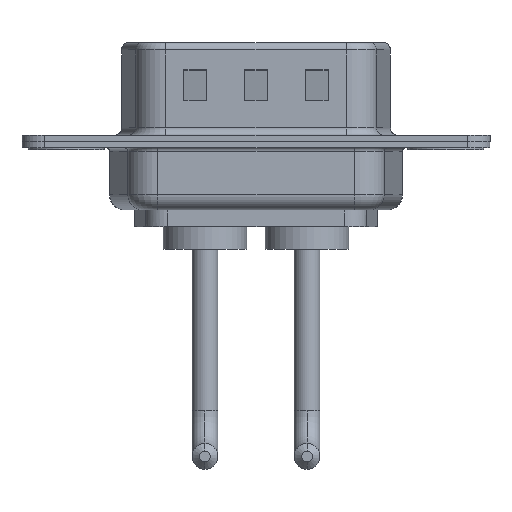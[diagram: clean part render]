
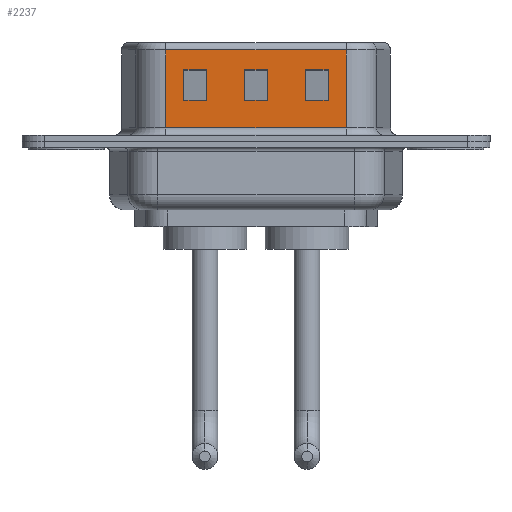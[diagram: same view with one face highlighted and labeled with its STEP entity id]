
A CAD part, front view. The second image highlights one B-rep face of the part: STEP entity #2237.
In plain terms, the highlighted planar face has unit normal (0, -1, 0).
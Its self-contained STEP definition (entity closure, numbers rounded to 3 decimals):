
#38 = VECTOR ( 'NONE', #927, 1000. ) ;
#124 = VERTEX_POINT ( 'NONE', #11989 ) ;
#233 = LINE ( 'NONE', #4109, #7689 ) ;
#274 = CARTESIAN_POINT ( 'NONE',  ( 22.451, -4.55, 2.705 ) ) ;
#290 = CARTESIAN_POINT ( 'NONE',  ( 18.451, -4.55, 6.52 ) ) ;
#459 = EDGE_CURVE ( 'NONE', #4935, #2185, #12560, .T. ) ;
#797 = VECTOR ( 'NONE', #11295, 1000. ) ;
#838 = ORIENTED_EDGE ( 'NONE', *, *, #1437, .T. ) ;
#859 = LINE ( 'NONE', #5694, #10427 ) ;
#927 = DIRECTION ( 'NONE',  ( -1., 0., 0. ) ) ;
#1058 = ORIENTED_EDGE ( 'NONE', *, *, #2612, .T. ) ;
#1204 = CARTESIAN_POINT ( 'NONE',  ( 18.451, -4.55, 6.52 ) ) ;
#1213 = DIRECTION ( 'NONE',  ( 0., 0., -1. ) ) ;
#1287 = DIRECTION ( 'NONE',  ( -1., 0., 0. ) ) ;
#1318 = VECTOR ( 'NONE', #7643, 1000. ) ;
#1386 = VECTOR ( 'NONE', #2738, 1000. ) ;
#1404 = EDGE_LOOP ( 'NONE', ( #4933, #6059, #4356, #838 ) ) ;
#1411 = EDGE_CURVE ( 'NONE', #7855, #5947, #2452, .T. ) ;
#1437 = EDGE_CURVE ( 'NONE', #5947, #4728, #233, .T. ) ;
#1714 = LINE ( 'NONE', #5466, #8401 ) ;
#1787 = CARTESIAN_POINT ( 'NONE',  ( 7.75, -4.55, 6.52 ) ) ;
#1921 = VECTOR ( 'NONE', #7525, 1000. ) ;
#1956 = ORIENTED_EDGE ( 'NONE', *, *, #8740, .T. ) ;
#2049 = CARTESIAN_POINT ( 'NONE',  ( 6.549, -4.55, 6.02 ) ) ;
#2185 = VERTEX_POINT ( 'NONE', #8154 ) ;
#2227 = CARTESIAN_POINT ( 'NONE',  ( 17.25, -4.55, 6.52 ) ) ;
#2237 = ADVANCED_FACE ( 'NONE', ( #4418, #5239, #2308, #10213 ), #10157, .F. ) ;
#2308 = FACE_BOUND ( 'NONE', #1404, .T. ) ;
#2369 = EDGE_CURVE ( 'NONE', #5578, #124, #2575, .T. ) ;
#2452 = LINE ( 'NONE', #5248, #5029 ) ;
#2552 = ORIENTED_EDGE ( 'NONE', *, *, #2369, .T. ) ;
#2575 = LINE ( 'NONE', #8352, #8101 ) ;
#2612 = EDGE_CURVE ( 'NONE', #11123, #5578, #9046, .T. ) ;
#2683 = DIRECTION ( 'NONE',  ( 1., 0., 0. ) ) ;
#2738 = DIRECTION ( 'NONE',  ( 0., 0., 1. ) ) ;
#2807 = CARTESIAN_POINT ( 'NONE',  ( 13.25, -4.55, 4.705 ) ) ;
#2811 = CARTESIAN_POINT ( 'NONE',  ( 7.75, -4.55, 4.705 ) ) ;
#3108 = LINE ( 'NONE', #1204, #11344 ) ;
#3168 = AXIS2_PLACEMENT_3D ( 'NONE', #290, #3390, #10022 ) ;
#3349 = DIRECTION ( 'NONE',  ( 1., 0., 0. ) ) ;
#3390 = DIRECTION ( 'NONE',  ( 0., 1., 0. ) ) ;
#3591 = VECTOR ( 'NONE', #3349, 1000. ) ;
#3698 = DIRECTION ( 'NONE',  ( 1., 0., 0. ) ) ;
#3762 = LINE ( 'NONE', #12538, #1318 ) ;
#3776 = CARTESIAN_POINT ( 'NONE',  ( 18.451, -4.55, 6.02 ) ) ;
#4065 = DIRECTION ( 'NONE',  ( 0., 0., -1. ) ) ;
#4109 = CARTESIAN_POINT ( 'NONE',  ( 11.75, -4.55, 6.52 ) ) ;
#4259 = LINE ( 'NONE', #2227, #9663 ) ;
#4319 = CARTESIAN_POINT ( 'NONE',  ( 18.451, -4.55, 0.9 ) ) ;
#4356 = ORIENTED_EDGE ( 'NONE', *, *, #1411, .T. ) ;
#4418 = FACE_BOUND ( 'NONE', #11009, .T. ) ;
#4422 = LINE ( 'NONE', #12182, #797 ) ;
#4488 = EDGE_CURVE ( 'NONE', #11314, #11445, #859, .T. ) ;
#4728 = VERTEX_POINT ( 'NONE', #6696 ) ;
#4814 = ORIENTED_EDGE ( 'NONE', *, *, #8811, .T. ) ;
#4822 = CARTESIAN_POINT ( 'NONE',  ( 15.75, -4.55, 2.705 ) ) ;
#4933 = ORIENTED_EDGE ( 'NONE', *, *, #6079, .T. ) ;
#4935 = VERTEX_POINT ( 'NONE', #10444 ) ;
#5029 = VECTOR ( 'NONE', #9069, 1000. ) ;
#5048 = VERTEX_POINT ( 'NONE', #8716 ) ;
#5154 = ORIENTED_EDGE ( 'NONE', *, *, #7612, .T. ) ;
#5190 = VERTEX_POINT ( 'NONE', #11044 ) ;
#5239 = FACE_BOUND ( 'NONE', #7296, .T. ) ;
#5248 = CARTESIAN_POINT ( 'NONE',  ( 18.451, -4.55, 2.705 ) ) ;
#5315 = EDGE_CURVE ( 'NONE', #8747, #7855, #1714, .T. ) ;
#5466 = CARTESIAN_POINT ( 'NONE',  ( 13.25, -4.55, 6.52 ) ) ;
#5544 = ORIENTED_EDGE ( 'NONE', *, *, #10372, .T. ) ;
#5578 = VERTEX_POINT ( 'NONE', #4822 ) ;
#5694 = CARTESIAN_POINT ( 'NONE',  ( 18.451, -4.55, 6.02 ) ) ;
#5728 = ORIENTED_EDGE ( 'NONE', *, *, #11827, .T. ) ;
#5752 = CARTESIAN_POINT ( 'NONE',  ( 14.451, -4.55, 2.705 ) ) ;
#5882 = VERTEX_POINT ( 'NONE', #11199 ) ;
#5947 = VERTEX_POINT ( 'NONE', #7461 ) ;
#6023 = VERTEX_POINT ( 'NONE', #2811 ) ;
#6059 = ORIENTED_EDGE ( 'NONE', *, *, #5315, .T. ) ;
#6079 = EDGE_CURVE ( 'NONE', #4728, #8747, #8773, .T. ) ;
#6341 = DIRECTION ( 'NONE',  ( 0., 0., -1. ) ) ;
#6696 = CARTESIAN_POINT ( 'NONE',  ( 11.75, -4.55, 4.705 ) ) ;
#6720 = ORIENTED_EDGE ( 'NONE', *, *, #459, .T. ) ;
#7069 = EDGE_LOOP ( 'NONE', ( #11879, #8375, #1956, #4814 ) ) ;
#7234 = EDGE_CURVE ( 'NONE', #5882, #4935, #11337, .T. ) ;
#7296 = EDGE_LOOP ( 'NONE', ( #5154, #1058, #2552, #5544 ) ) ;
#7461 = CARTESIAN_POINT ( 'NONE',  ( 11.75, -4.55, 2.705 ) ) ;
#7525 = DIRECTION ( 'NONE',  ( 0., 0., -1. ) ) ;
#7581 = VECTOR ( 'NONE', #2683, 1000. ) ;
#7612 = EDGE_CURVE ( 'NONE', #5190, #11123, #4259, .T. ) ;
#7643 = DIRECTION ( 'NONE',  ( 0., 0., -1. ) ) ;
#7689 = VECTOR ( 'NONE', #10292, 1000. ) ;
#7739 = VERTEX_POINT ( 'NONE', #4319 ) ;
#7817 = VECTOR ( 'NONE', #3698, 1000. ) ;
#7855 = VERTEX_POINT ( 'NONE', #8141 ) ;
#8101 = VECTOR ( 'NONE', #12242, 1000. ) ;
#8141 = CARTESIAN_POINT ( 'NONE',  ( 13.25, -4.55, 2.705 ) ) ;
#8154 = CARTESIAN_POINT ( 'NONE',  ( 7.75, -4.55, 2.705 ) ) ;
#8180 = CARTESIAN_POINT ( 'NONE',  ( 22.451, -4.55, 4.705 ) ) ;
#8352 = CARTESIAN_POINT ( 'NONE',  ( 15.75, -4.55, 6.52 ) ) ;
#8375 = ORIENTED_EDGE ( 'NONE', *, *, #4488, .T. ) ;
#8401 = VECTOR ( 'NONE', #6341, 1000. ) ;
#8417 = DIRECTION ( 'NONE',  ( -1., 0., 0. ) ) ;
#8662 = ORIENTED_EDGE ( 'NONE', *, *, #7234, .T. ) ;
#8716 = CARTESIAN_POINT ( 'NONE',  ( 6.549, -4.55, 0.9 ) ) ;
#8740 = EDGE_CURVE ( 'NONE', #11445, #5048, #3762, .T. ) ;
#8747 = VERTEX_POINT ( 'NONE', #2807 ) ;
#8773 = LINE ( 'NONE', #11644, #7581 ) ;
#8811 = EDGE_CURVE ( 'NONE', #5048, #7739, #10445, .T. ) ;
#9046 = LINE ( 'NONE', #274, #12534 ) ;
#9069 = DIRECTION ( 'NONE',  ( -1., 0., 0. ) ) ;
#9511 = CARTESIAN_POINT ( 'NONE',  ( 18.451, -4.55, 0.9 ) ) ;
#9623 = LINE ( 'NONE', #1787, #1386 ) ;
#9663 = VECTOR ( 'NONE', #1213, 1000. ) ;
#10022 = DIRECTION ( 'NONE',  ( -1., 0., 0. ) ) ;
#10049 = LINE ( 'NONE', #8180, #3591 ) ;
#10157 = PLANE ( 'NONE',  #3168 ) ;
#10213 = FACE_OUTER_BOUND ( 'NONE', #7069, .T. ) ;
#10292 = DIRECTION ( 'NONE',  ( 0., 0., 1. ) ) ;
#10372 = EDGE_CURVE ( 'NONE', #124, #5190, #10049, .T. ) ;
#10427 = VECTOR ( 'NONE', #8417, 1000. ) ;
#10444 = CARTESIAN_POINT ( 'NONE',  ( 9.25, -4.55, 2.705 ) ) ;
#10445 = LINE ( 'NONE', #9511, #7817 ) ;
#10828 = CARTESIAN_POINT ( 'NONE',  ( 17.25, -4.55, 2.705 ) ) ;
#10950 = ORIENTED_EDGE ( 'NONE', *, *, #12001, .T. ) ;
#11009 = EDGE_LOOP ( 'NONE', ( #8662, #6720, #5728, #10950 ) ) ;
#11044 = CARTESIAN_POINT ( 'NONE',  ( 17.25, -4.55, 4.705 ) ) ;
#11123 = VERTEX_POINT ( 'NONE', #10828 ) ;
#11199 = CARTESIAN_POINT ( 'NONE',  ( 9.25, -4.55, 4.705 ) ) ;
#11202 = CARTESIAN_POINT ( 'NONE',  ( 9.25, -4.55, 6.52 ) ) ;
#11295 = DIRECTION ( 'NONE',  ( 1., 0., 0. ) ) ;
#11314 = VERTEX_POINT ( 'NONE', #3776 ) ;
#11337 = LINE ( 'NONE', #11202, #1921 ) ;
#11344 = VECTOR ( 'NONE', #4065, 1000. ) ;
#11445 = VERTEX_POINT ( 'NONE', #2049 ) ;
#11644 = CARTESIAN_POINT ( 'NONE',  ( 18.451, -4.55, 4.705 ) ) ;
#11827 = EDGE_CURVE ( 'NONE', #2185, #6023, #9623, .T. ) ;
#11879 = ORIENTED_EDGE ( 'NONE', *, *, #11957, .F. ) ;
#11957 = EDGE_CURVE ( 'NONE', #11314, #7739, #3108, .T. ) ;
#11989 = CARTESIAN_POINT ( 'NONE',  ( 15.75, -4.55, 4.705 ) ) ;
#12001 = EDGE_CURVE ( 'NONE', #6023, #5882, #4422, .T. ) ;
#12182 = CARTESIAN_POINT ( 'NONE',  ( 14.451, -4.55, 4.705 ) ) ;
#12242 = DIRECTION ( 'NONE',  ( 0., 0., 1. ) ) ;
#12534 = VECTOR ( 'NONE', #1287, 1000. ) ;
#12538 = CARTESIAN_POINT ( 'NONE',  ( 6.549, -4.55, 6.52 ) ) ;
#12560 = LINE ( 'NONE', #5752, #38 ) ;
